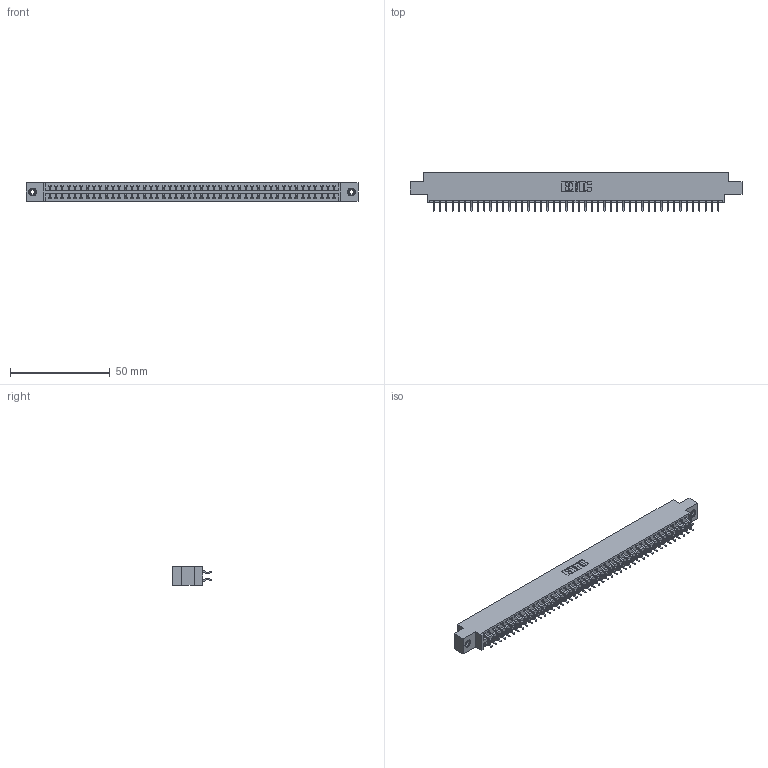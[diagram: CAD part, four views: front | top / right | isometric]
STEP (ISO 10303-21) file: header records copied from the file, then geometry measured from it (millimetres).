
FILE_DESCRIPTION (( 'STEP AP203' ), '1' );
FILE_NAME ('346-092-556-808.STEP', '2022-05-26T08:05:42', ( '' ), ( '' ), 'SwSTEP 2.0', 'SolidWorks 2020', '' );
FILE_SCHEMA (( 'CONFIG_CONTROL_DESIGN' ));
Length unit declared in the file: inch
Products named in the file (4): 345-250-001_345-250-003-102; 345-292-001_556 Tail; 346-092-556-808; 346 Part_0.170 Offset - 0.156 Dia-TI
Assembly tree (95 placements, depth 2):
  346-092-556-808
    346 Part_0.170 Offset - 0.156 Dia-TI
    345-292-001_556 Tail  x92
    345-250-001_345-250-003-102  x2
Bounding box: 166.62 x 19.57 x 9.4 mm (x, y, z)
Volume: 16114.2 mm3; surface area: 22327.1 mm2
Topology: 95 solids, 95 shells, 5522 faces, 16393 edges, 10798 vertices
Faces by surface type: plane 3700, cylinder 1806, cone 12, torus 4
Entity records: 31020 total; most frequent: CARTESIAN_POINT 5107, ORIENTED_EDGE 5022, DIRECTION 4565, EDGE_CURVE 2511, LINE 2167, VECTOR 2167, VERTEX_POINT 1668, AXIS2_PLACEMENT_3D 1199
